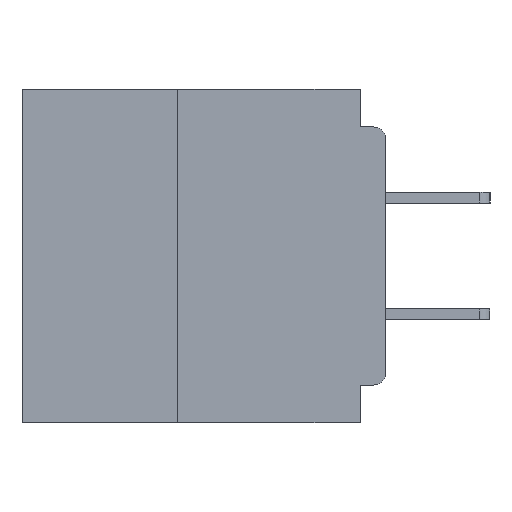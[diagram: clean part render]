
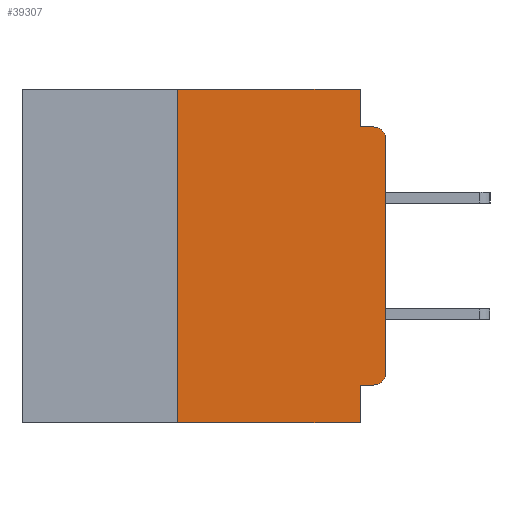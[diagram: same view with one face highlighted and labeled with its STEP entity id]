
A CAD part, left-side view. The second image highlights one B-rep face of the part: STEP entity #39307.
In plain terms, the highlighted planar face has unit normal (-1, 0, 0).
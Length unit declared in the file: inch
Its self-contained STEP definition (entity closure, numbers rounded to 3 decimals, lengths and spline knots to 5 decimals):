
#608 = AXIS2_PLACEMENT_3D ( 'NONE', #38505, #19109, #41709 ) ;
#756 = EDGE_CURVE ( 'NONE', #37666, #23789, #10080, .T. ) ;
#1358 = LINE ( 'NONE', #30734, #27485 ) ;
#1970 = DIRECTION ( 'NONE',  ( 0., -1., 0. ) ) ;
#2575 = CARTESIAN_POINT ( 'NONE',  ( 0., 0.25, -0.4 ) ) ;
#2874 = CARTESIAN_POINT ( 'NONE',  ( 0., 0., -0.06 ) ) ;
#4042 = DIRECTION ( 'NONE',  ( 0., 0., 1. ) ) ;
#4116 = LINE ( 'NONE', #24890, #12906 ) ;
#4601 = DIRECTION ( 'NONE',  ( 0., 1., 0. ) ) ;
#4732 = DIRECTION ( 'NONE',  ( 1., 0., 0. ) ) ;
#4788 = VERTEX_POINT ( 'NONE', #9806 ) ;
#6410 = CARTESIAN_POINT ( 'NONE',  ( 0., 0., 0. ) ) ;
#6653 = CIRCLE ( 'NONE', #27888, 0.015 ) ;
#7299 = ORIENTED_EDGE ( 'NONE', *, *, #34227, .T. ) ;
#7328 = VECTOR ( 'NONE', #21618, 39.37008 ) ;
#8847 = EDGE_CURVE ( 'NONE', #4788, #26512, #41806, .T. ) ;
#9343 = EDGE_CURVE ( 'NONE', #17583, #26933, #40760, .T. ) ;
#9806 = CARTESIAN_POINT ( 'NONE',  ( 0., 0.031, 0. ) ) ;
#10080 = LINE ( 'NONE', #2575, #19752 ) ;
#10466 = LINE ( 'NONE', #15536, #17109 ) ;
#11074 = DIRECTION ( 'NONE',  ( 0., 0., -1. ) ) ;
#11376 = VERTEX_POINT ( 'NONE', #38514 ) ;
#11593 = CARTESIAN_POINT ( 'NONE',  ( 0., 0.015, -0.06 ) ) ;
#12399 = AXIS2_PLACEMENT_3D ( 'NONE', #37219, #4732, #27585 ) ;
#12699 = VERTEX_POINT ( 'NONE', #23026 ) ;
#12906 = VECTOR ( 'NONE', #1970, 39.37008 ) ;
#13889 = VERTEX_POINT ( 'NONE', #34695 ) ;
#13961 = EDGE_CURVE ( 'NONE', #23789, #4788, #10466, .T. ) ;
#13964 = ORIENTED_EDGE ( 'NONE', *, *, #29686, .F. ) ;
#14388 = CARTESIAN_POINT ( 'NONE',  ( 0., 0.25, 0. ) ) ;
#14875 = DIRECTION ( 'NONE',  ( 0., 0., -1. ) ) ;
#15536 = CARTESIAN_POINT ( 'NONE',  ( 0., 0.437, 0. ) ) ;
#17109 = VECTOR ( 'NONE', #18779, 39.37008 ) ;
#17583 = VERTEX_POINT ( 'NONE', #39457 ) ;
#18362 = CARTESIAN_POINT ( 'NONE',  ( 0., 0.031, 0. ) ) ;
#18779 = DIRECTION ( 'NONE',  ( 0., -1., 0. ) ) ;
#18825 = EDGE_CURVE ( 'NONE', #11376, #23484, #33931, .T. ) ;
#19109 = DIRECTION ( 'NONE',  ( -1., 0., 0. ) ) ;
#19533 = ORIENTED_EDGE ( 'NONE', *, *, #756, .F. ) ;
#19546 = CARTESIAN_POINT ( 'NONE',  ( 0., 0.031, -0.4 ) ) ;
#19752 = VECTOR ( 'NONE', #4042, 39.37008 ) ;
#21618 = DIRECTION ( 'NONE',  ( 0., 0., -1. ) ) ;
#23026 = CARTESIAN_POINT ( 'NONE',  ( 0., 0.015, -0.045 ) ) ;
#23082 = ORIENTED_EDGE ( 'NONE', *, *, #29122, .T. ) ;
#23484 = VERTEX_POINT ( 'NONE', #2874 ) ;
#23578 = VECTOR ( 'NONE', #11074, 39.37008 ) ;
#23789 = VERTEX_POINT ( 'NONE', #14388 ) ;
#23810 = CARTESIAN_POINT ( 'NONE',  ( 0., 0.031, -0.045 ) ) ;
#24304 = PLANE ( 'NONE',  #12399 ) ;
#24789 = LINE ( 'NONE', #37431, #40951 ) ;
#24890 = CARTESIAN_POINT ( 'NONE',  ( 0., 0.437, -0.4 ) ) ;
#26123 = ORIENTED_EDGE ( 'NONE', *, *, #8847, .F. ) ;
#26512 = VERTEX_POINT ( 'NONE', #23810 ) ;
#26933 = VERTEX_POINT ( 'NONE', #19546 ) ;
#27344 = EDGE_CURVE ( 'NONE', #37666, #26933, #4116, .T. ) ;
#27485 = VECTOR ( 'NONE', #4601, 39.37008 ) ;
#27585 = DIRECTION ( 'NONE',  ( 0., 0., -1. ) ) ;
#27888 = AXIS2_PLACEMENT_3D ( 'NONE', #11593, #34337, #14875 ) ;
#27904 = CARTESIAN_POINT ( 'NONE',  ( 0., 0.25, -0.4 ) ) ;
#29122 = EDGE_CURVE ( 'NONE', #23484, #12699, #6653, .T. ) ;
#29686 = EDGE_CURVE ( 'NONE', #13889, #17583, #1358, .T. ) ;
#30734 = CARTESIAN_POINT ( 'NONE',  ( 0., 0., -0.355 ) ) ;
#30947 = DIRECTION ( 'NONE',  ( 0., -1., 0. ) ) ;
#33931 = LINE ( 'NONE', #6410, #41414 ) ;
#34227 = EDGE_CURVE ( 'NONE', #13889, #11376, #41724, .T. ) ;
#34337 = DIRECTION ( 'NONE',  ( -1., 0., 0. ) ) ;
#34441 = FACE_OUTER_BOUND ( 'NONE', #37423, .T. ) ;
#34695 = CARTESIAN_POINT ( 'NONE',  ( 0., 0.015, -0.355 ) ) ;
#34776 = ORIENTED_EDGE ( 'NONE', *, *, #13961, .F. ) ;
#35731 = DIRECTION ( 'NONE',  ( 0., 0., 1. ) ) ;
#36787 = CARTESIAN_POINT ( 'NONE',  ( 0., 0.031, -0.4 ) ) ;
#36792 = ORIENTED_EDGE ( 'NONE', *, *, #27344, .T. ) ;
#37219 = CARTESIAN_POINT ( 'NONE',  ( 0., 0.437, 0. ) ) ;
#37423 = EDGE_LOOP ( 'NONE', ( #38246, #23082, #40270, #26123, #34776, #19533, #36792, #38776, #13964, #7299 ) ) ;
#37431 = CARTESIAN_POINT ( 'NONE',  ( 0., 0., -0.045 ) ) ;
#37666 = VERTEX_POINT ( 'NONE', #27904 ) ;
#38246 = ORIENTED_EDGE ( 'NONE', *, *, #18825, .T. ) ;
#38505 = CARTESIAN_POINT ( 'NONE',  ( 0., 0.015, -0.34 ) ) ;
#38514 = CARTESIAN_POINT ( 'NONE',  ( 0., 0., -0.34 ) ) ;
#38776 = ORIENTED_EDGE ( 'NONE', *, *, #9343, .F. ) ;
#38936 = EDGE_CURVE ( 'NONE', #26512, #12699, #24789, .T. ) ;
#39307 = ADVANCED_FACE ( 'NONE', ( #34441 ), #24304, .F. ) ;
#39457 = CARTESIAN_POINT ( 'NONE',  ( 0., 0.031, -0.355 ) ) ;
#40270 = ORIENTED_EDGE ( 'NONE', *, *, #38936, .F. ) ;
#40760 = LINE ( 'NONE', #36787, #23578 ) ;
#40951 = VECTOR ( 'NONE', #30947, 39.37008 ) ;
#41414 = VECTOR ( 'NONE', #35731, 39.37008 ) ;
#41709 = DIRECTION ( 'NONE',  ( 0., 0., -1. ) ) ;
#41724 = CIRCLE ( 'NONE', #608, 0.015 ) ;
#41806 = LINE ( 'NONE', #18362, #7328 ) ;
